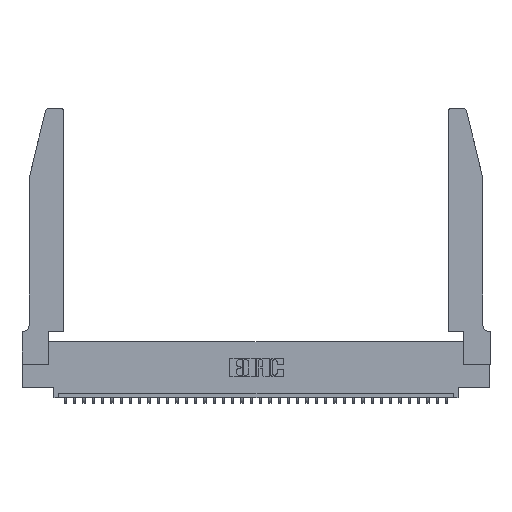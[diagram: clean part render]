
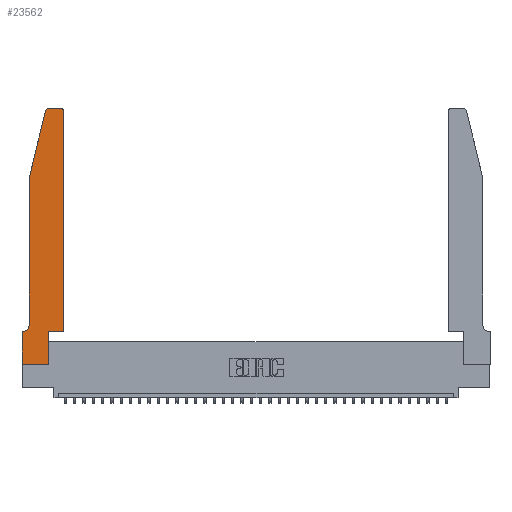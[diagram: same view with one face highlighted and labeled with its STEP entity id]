
A CAD part, top view. The second image highlights one B-rep face of the part: STEP entity #23562.
In plain terms, the highlighted planar face has unit normal (0, 0, 1).
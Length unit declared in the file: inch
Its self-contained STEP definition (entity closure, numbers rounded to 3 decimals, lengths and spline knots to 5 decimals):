
#65 = LINE ( 'NONE', #9195, #18949 ) ;
#427 = ORIENTED_EDGE ( 'NONE', *, *, #4903, .T. ) ;
#516 = EDGE_CURVE ( 'NONE', #12048, #17353, #35960, .T. ) ;
#522 = VERTEX_POINT ( 'NONE', #19120 ) ;
#911 = DIRECTION ( 'NONE',  ( 0., 1., 0. ) ) ;
#1584 = CARTESIAN_POINT ( 'NONE',  ( 0.4505, 0.35, 0.37 ) ) ;
#2423 = CARTESIAN_POINT ( 'NONE',  ( 0.4205, 2.72, 0.37 ) ) ;
#2526 = EDGE_CURVE ( 'NONE', #36326, #33570, #65, .T. ) ;
#2595 = EDGE_CURVE ( 'NONE', #34419, #25821, #27365, .T. ) ;
#2855 = CARTESIAN_POINT ( 'NONE',  ( 0., 0.35, 0.37 ) ) ;
#2979 = VECTOR ( 'NONE', #34997, 39.37008 ) ;
#3365 = ORIENTED_EDGE ( 'NONE', *, *, #3447, .T. ) ;
#3447 = EDGE_CURVE ( 'NONE', #13313, #36326, #34218, .T. ) ;
#4483 = ORIENTED_EDGE ( 'NONE', *, *, #20409, .T. ) ;
#4834 = CARTESIAN_POINT ( 'NONE',  ( 0.0055, 0.35, 0.37 ) ) ;
#4903 = EDGE_CURVE ( 'NONE', #20669, #13313, #34621, .T. ) ;
#5487 = EDGE_CURVE ( 'NONE', #30189, #522, #35520, .T. ) ;
#6507 = DIRECTION ( 'NONE',  ( 0., -1., 0. ) ) ;
#7219 = CARTESIAN_POINT ( 'NONE',  ( 0.4505, 2.72, 0.37 ) ) ;
#7655 = VECTOR ( 'NONE', #9170, 39.37008 ) ;
#8357 = EDGE_CURVE ( 'NONE', #33570, #34419, #13077, .T. ) ;
#8362 = CARTESIAN_POINT ( 'NONE',  ( 0.0755, 2., 0.37 ) ) ;
#8569 = VERTEX_POINT ( 'NONE', #28561 ) ;
#8710 = CARTESIAN_POINT ( 'NONE',  ( 0.284, 2.75, 0.37 ) ) ;
#9170 = DIRECTION ( 'NONE',  ( 0., 1., 0. ) ) ;
#9195 = CARTESIAN_POINT ( 'NONE',  ( 0.0755, 2., 0.37 ) ) ;
#11160 = EDGE_CURVE ( 'NONE', #17353, #8569, #29302, .T. ) ;
#12048 = VERTEX_POINT ( 'NONE', #1584 ) ;
#12146 = LINE ( 'NONE', #32115, #2979 ) ;
#12162 = ORIENTED_EDGE ( 'NONE', *, *, #2595, .T. ) ;
#12301 = VECTOR ( 'NONE', #31011, 39.37008 ) ;
#12387 = CARTESIAN_POINT ( 'NONE',  ( 0., 0., 0.37 ) ) ;
#12423 = VECTOR ( 'NONE', #14237, 39.37008 ) ;
#12919 = DIRECTION ( 'NONE',  ( 0., 0., 1. ) ) ;
#13077 = CIRCLE ( 'NONE', #36378, 0.07 ) ;
#13313 = VERTEX_POINT ( 'NONE', #17604 ) ;
#13734 = AXIS2_PLACEMENT_3D ( 'NONE', #29331, #24148, #32348 ) ;
#14008 = EDGE_CURVE ( 'NONE', #522, #18779, #31787, .T. ) ;
#14113 = EDGE_LOOP ( 'NONE', ( #17375, #427, #3365, #33220, #30909, #12162, #30046, #23368, #18057, #4483, #29560, #17234 ) ) ;
#14237 = DIRECTION ( 'NONE',  ( 1., 0., 0. ) ) ;
#14995 = VECTOR ( 'NONE', #17442, 39.37008 ) ;
#15332 = CARTESIAN_POINT ( 'NONE',  ( 0.2865, 0.35, 0.37 ) ) ;
#16171 = DIRECTION ( 'NONE',  ( 1., 0., 0. ) ) ;
#16549 = DIRECTION ( 'NONE',  ( 0., 0., 1. ) ) ;
#16874 = FACE_OUTER_BOUND ( 'NONE', #14113, .T. ) ;
#17137 = AXIS2_PLACEMENT_3D ( 'NONE', #33087, #12919, #16171 ) ;
#17234 = ORIENTED_EDGE ( 'NONE', *, *, #11160, .T. ) ;
#17353 = VERTEX_POINT ( 'NONE', #7219 ) ;
#17375 = ORIENTED_EDGE ( 'NONE', *, *, #28345, .T. ) ;
#17442 = DIRECTION ( 'NONE',  ( 0., -1., 0. ) ) ;
#17518 = LINE ( 'NONE', #28549, #26380 ) ;
#17604 = CARTESIAN_POINT ( 'NONE',  ( 0.25487, 2.72718, 0.37 ) ) ;
#17640 = LINE ( 'NONE', #12387, #14995 ) ;
#18057 = ORIENTED_EDGE ( 'NONE', *, *, #14008, .T. ) ;
#18779 = VERTEX_POINT ( 'NONE', #15332 ) ;
#18949 = VECTOR ( 'NONE', #6507, 39.37008 ) ;
#19120 = CARTESIAN_POINT ( 'NONE',  ( 0.2865, 0., 0.37 ) ) ;
#19286 = DIRECTION ( 'NONE',  ( -0.239, -0.971, 0. ) ) ;
#19349 = DIRECTION ( 'NONE',  ( 1., 0., 0. ) ) ;
#20409 = EDGE_CURVE ( 'NONE', #18779, #12048, #17518, .T. ) ;
#20669 = VERTEX_POINT ( 'NONE', #8710 ) ;
#21438 = PLANE ( 'NONE',  #17137 ) ;
#22384 = CARTESIAN_POINT ( 'NONE',  ( 0., 0., 0.37 ) ) ;
#22893 = CARTESIAN_POINT ( 'NONE',  ( 0., 0., 0.37 ) ) ;
#22978 = DIRECTION ( 'NONE',  ( 1., 0., 0. ) ) ;
#23368 = ORIENTED_EDGE ( 'NONE', *, *, #5487, .T. ) ;
#23414 = CARTESIAN_POINT ( 'NONE',  ( 0.0055, 0.42, 0.37 ) ) ;
#23562 = ADVANCED_FACE ( 'NONE', ( #16874 ), #21438, .T. ) ;
#23795 = CARTESIAN_POINT ( 'NONE',  ( 0.0755, 0.42, 0.37 ) ) ;
#23814 = CARTESIAN_POINT ( 'NONE',  ( 0.0755, 2., 0.37 ) ) ;
#24066 = EDGE_CURVE ( 'NONE', #25821, #30189, #17640, .T. ) ;
#24148 = DIRECTION ( 'NONE',  ( 0., 0., 1. ) ) ;
#25454 = CARTESIAN_POINT ( 'NONE',  ( 0.0755, 0.35, 0.37 ) ) ;
#25821 = VERTEX_POINT ( 'NONE', #2855 ) ;
#26271 = DIRECTION ( 'NONE',  ( -1., 0., 0. ) ) ;
#26380 = VECTOR ( 'NONE', #22978, 39.37008 ) ;
#27365 = LINE ( 'NONE', #25454, #12301 ) ;
#28345 = EDGE_CURVE ( 'NONE', #8569, #20669, #12146, .T. ) ;
#28549 = CARTESIAN_POINT ( 'NONE',  ( 0.4505, 0.35, 0.37 ) ) ;
#28561 = CARTESIAN_POINT ( 'NONE',  ( 0.4205, 2.75, 0.37 ) ) ;
#29227 = DIRECTION ( 'NONE',  ( 0., 0., -1. ) ) ;
#29302 = CIRCLE ( 'NONE', #33771, 0.03 ) ;
#29331 = CARTESIAN_POINT ( 'NONE',  ( 0.284, 2.72, 0.37 ) ) ;
#29560 = ORIENTED_EDGE ( 'NONE', *, *, #516, .T. ) ;
#30046 = ORIENTED_EDGE ( 'NONE', *, *, #24066, .T. ) ;
#30189 = VERTEX_POINT ( 'NONE', #22893 ) ;
#30909 = ORIENTED_EDGE ( 'NONE', *, *, #8357, .T. ) ;
#31011 = DIRECTION ( 'NONE',  ( -1., 0., 0. ) ) ;
#31787 = LINE ( 'NONE', #34707, #33589 ) ;
#32115 = CARTESIAN_POINT ( 'NONE',  ( 0.2605, 2.75, 0.37 ) ) ;
#32348 = DIRECTION ( 'NONE',  ( 1., 0., 0. ) ) ;
#33087 = CARTESIAN_POINT ( 'NONE',  ( 0., 0.35, 0.37 ) ) ;
#33220 = ORIENTED_EDGE ( 'NONE', *, *, #2526, .T. ) ;
#33344 = VECTOR ( 'NONE', #19286, 39.37008 ) ;
#33570 = VERTEX_POINT ( 'NONE', #23795 ) ;
#33589 = VECTOR ( 'NONE', #911, 39.37008 ) ;
#33771 = AXIS2_PLACEMENT_3D ( 'NONE', #2423, #16549, #19349 ) ;
#34218 = LINE ( 'NONE', #8362, #33344 ) ;
#34419 = VERTEX_POINT ( 'NONE', #4834 ) ;
#34621 = CIRCLE ( 'NONE', #13734, 0.03 ) ;
#34707 = CARTESIAN_POINT ( 'NONE',  ( 0.2865, 0.35, 0.37 ) ) ;
#34997 = DIRECTION ( 'NONE',  ( -1., 0., 0. ) ) ;
#35132 = CARTESIAN_POINT ( 'NONE',  ( 0.4505, 0.35, 0.37 ) ) ;
#35520 = LINE ( 'NONE', #22384, #12423 ) ;
#35960 = LINE ( 'NONE', #35132, #7655 ) ;
#36326 = VERTEX_POINT ( 'NONE', #23814 ) ;
#36378 = AXIS2_PLACEMENT_3D ( 'NONE', #23414, #29227, #26271 ) ;
